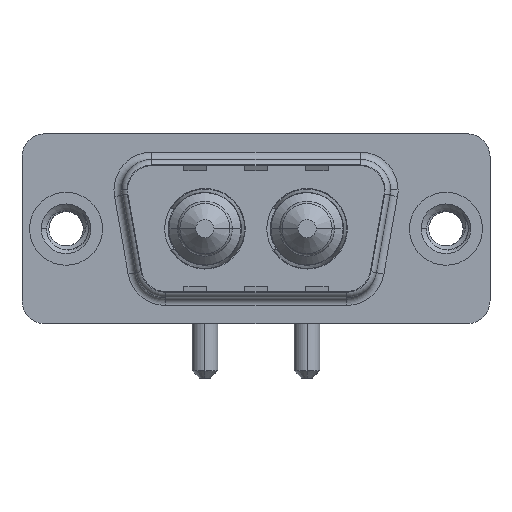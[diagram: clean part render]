
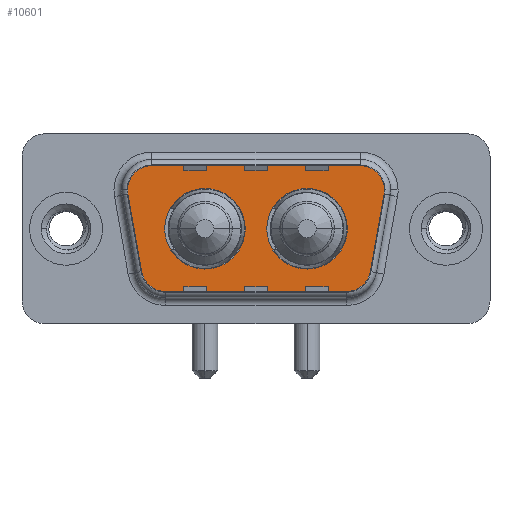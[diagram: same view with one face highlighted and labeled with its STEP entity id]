
A CAD part, top view. The second image highlights one B-rep face of the part: STEP entity #10601.
In plain terms, the highlighted planar face has unit normal (0, 0, 1).
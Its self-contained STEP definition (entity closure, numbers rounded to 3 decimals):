
#121 = EDGE_CURVE ( 'NONE', #11230, #8810, #10595, .T. ) ;
#185 = DIRECTION ( 'NONE',  ( 0., 0., 1. ) ) ;
#381 = DIRECTION ( 'NONE',  ( 0., 0., 1. ) ) ;
#634 = CARTESIAN_POINT ( 'NONE',  ( 21.534, 2.553, 0. ) ) ;
#751 = VECTOR ( 'NONE', #9647, 1000. ) ;
#845 = ORIENTED_EDGE ( 'NONE', *, *, #121, .T. ) ;
#1028 = DIRECTION ( 'NONE',  ( 0., 0., 1. ) ) ;
#1068 = DIRECTION ( 'NONE',  ( 0., 0., 1. ) ) ;
#1150 = FACE_OUTER_BOUND ( 'NONE', #7707, .T. ) ;
#1158 = EDGE_CURVE ( 'NONE', #3391, #4372, #2509, .T. ) ;
#1253 = CARTESIAN_POINT ( 'NONE',  ( 5.436, 4.9, 0. ) ) ;
#1506 = DIRECTION ( 'NONE',  ( 0., 0., 1. ) ) ;
#1563 = CARTESIAN_POINT ( 'NONE',  ( 6.459, -2.9, 0. ) ) ;
#1573 = AXIS2_PLACEMENT_3D ( 'NONE', #2389, #1506, #6002 ) ;
#1911 = PLANE ( 'NONE',  #5977 ) ;
#1923 = EDGE_CURVE ( 'NONE', #4514, #3446, #9788, .T. ) ;
#2010 = EDGE_CURVE ( 'NONE', #5898, #9227, #8078, .T. ) ;
#2159 = CARTESIAN_POINT ( 'NONE',  ( 3.466, 2.553, 0. ) ) ;
#2242 = DIRECTION ( 'NONE',  ( 1., 0., 0. ) ) ;
#2358 = CARTESIAN_POINT ( 'NONE',  ( 9.14, 0., 0. ) ) ;
#2389 = CARTESIAN_POINT ( 'NONE',  ( 5.436, 2.9, 0. ) ) ;
#2408 = CARTESIAN_POINT ( 'NONE',  ( 21.564, 2.9, 0. ) ) ;
#2444 = ORIENTED_EDGE ( 'NONE', *, *, #6426, .T. ) ;
#2509 = LINE ( 'NONE', #634, #9070 ) ;
#2644 = CARTESIAN_POINT ( 'NONE',  ( 20.511, -3.247, 0. ) ) ;
#2742 = ORIENTED_EDGE ( 'NONE', *, *, #4454, .T. ) ;
#2781 = CARTESIAN_POINT ( 'NONE',  ( 3.466, 2.553, 0. ) ) ;
#2819 = CIRCLE ( 'NONE', #6562, 2.65 ) ;
#3036 = DIRECTION ( 'NONE',  ( 0.174, -0.985, 0. ) ) ;
#3181 = DIRECTION ( 'NONE',  ( 1., 0., 0. ) ) ;
#3182 = DIRECTION ( 'NONE',  ( -1., 0., 0. ) ) ;
#3293 = CARTESIAN_POINT ( 'NONE',  ( 18.541, -2.9, 0. ) ) ;
#3391 = VERTEX_POINT ( 'NONE', #2644 ) ;
#3446 = VERTEX_POINT ( 'NONE', #7868 ) ;
#3484 = CARTESIAN_POINT ( 'NONE',  ( 13.21, 0., 0. ) ) ;
#3557 = CIRCLE ( 'NONE', #7702, 2. ) ;
#4012 = CARTESIAN_POINT ( 'NONE',  ( 5.436, 4.9, 0. ) ) ;
#4174 = CARTESIAN_POINT ( 'NONE',  ( 19.564, 2.9, 0. ) ) ;
#4320 = DIRECTION ( 'NONE',  ( -1., 0., 0. ) ) ;
#4372 = VERTEX_POINT ( 'NONE', #6776 ) ;
#4383 = AXIS2_PLACEMENT_3D ( 'NONE', #1563, #1068, #4320 ) ;
#4435 = ORIENTED_EDGE ( 'NONE', *, *, #5691, .F. ) ;
#4448 = ORIENTED_EDGE ( 'NONE', *, *, #1923, .F. ) ;
#4454 = EDGE_CURVE ( 'NONE', #8600, #9421, #6631, .T. ) ;
#4482 = VECTOR ( 'NONE', #3036, 1000. ) ;
#4514 = VERTEX_POINT ( 'NONE', #3484 ) ;
#4700 = AXIS2_PLACEMENT_3D ( 'NONE', #2358, #5804, #2242 ) ;
#4724 = DIRECTION ( 'NONE',  ( 1., 0., 0. ) ) ;
#4771 = VERTEX_POINT ( 'NONE', #6532 ) ;
#4887 = DIRECTION ( 'NONE',  ( -1., 0., 0. ) ) ;
#4957 = LINE ( 'NONE', #2159, #4482 ) ;
#5174 = CARTESIAN_POINT ( 'NONE',  ( 19.564, 2.9, 0. ) ) ;
#5418 = VERTEX_POINT ( 'NONE', #5915 ) ;
#5480 = CARTESIAN_POINT ( 'NONE',  ( 18.541, -2.9, 0. ) ) ;
#5557 = ORIENTED_EDGE ( 'NONE', *, *, #11087, .F. ) ;
#5569 = DIRECTION ( 'NONE',  ( 1., 0., 0. ) ) ;
#5691 = EDGE_CURVE ( 'NONE', #9227, #5898, #7757, .T. ) ;
#5804 = DIRECTION ( 'NONE',  ( 0., 0., 1. ) ) ;
#5850 = CARTESIAN_POINT ( 'NONE',  ( 9.14, 0., 0. ) ) ;
#5898 = VERTEX_POINT ( 'NONE', #6249 ) ;
#5915 = CARTESIAN_POINT ( 'NONE',  ( 6.459, -4.9, 0. ) ) ;
#5937 = ORIENTED_EDGE ( 'NONE', *, *, #10634, .T. ) ;
#5977 = AXIS2_PLACEMENT_3D ( 'NONE', #5480, #1028, #4724 ) ;
#6002 = DIRECTION ( 'NONE',  ( 1., 0., 0. ) ) ;
#6005 = CARTESIAN_POINT ( 'NONE',  ( 11.79, 0., 0. ) ) ;
#6045 = CARTESIAN_POINT ( 'NONE',  ( 6.459, -4.9, 0. ) ) ;
#6171 = DIRECTION ( 'NONE',  ( 0., 0., 1. ) ) ;
#6249 = CARTESIAN_POINT ( 'NONE',  ( 6.49, 0., 0. ) ) ;
#6351 = FACE_BOUND ( 'NONE', #9599, .T. ) ;
#6426 = EDGE_CURVE ( 'NONE', #4771, #5418, #10391, .T. ) ;
#6454 = EDGE_CURVE ( 'NONE', #8810, #8600, #10176, .T. ) ;
#6532 = CARTESIAN_POINT ( 'NONE',  ( 4.489, -3.247, 0. ) ) ;
#6562 = AXIS2_PLACEMENT_3D ( 'NONE', #7341, #185, #5569 ) ;
#6631 = CIRCLE ( 'NONE', #1573, 2. ) ;
#6776 = CARTESIAN_POINT ( 'NONE',  ( 21.534, 2.553, 0. ) ) ;
#6900 = CIRCLE ( 'NONE', #11585, 2. ) ;
#7223 = CARTESIAN_POINT ( 'NONE',  ( 15.86, 0., 0. ) ) ;
#7251 = ORIENTED_EDGE ( 'NONE', *, *, #6454, .T. ) ;
#7341 = CARTESIAN_POINT ( 'NONE',  ( 15.86, 0., 0. ) ) ;
#7610 = CARTESIAN_POINT ( 'NONE',  ( 18.541, -4.9, 0. ) ) ;
#7702 = AXIS2_PLACEMENT_3D ( 'NONE', #3293, #381, #3181 ) ;
#7707 = EDGE_LOOP ( 'NONE', ( #8492, #11196, #10818, #845, #7251, #2742, #5937, #2444, #8847 ) ) ;
#7709 = DIRECTION ( 'NONE',  ( 0., 0., 1. ) ) ;
#7732 = AXIS2_PLACEMENT_3D ( 'NONE', #7223, #6171, #10755 ) ;
#7757 = CIRCLE ( 'NONE', #11485, 2.65 ) ;
#7868 = CARTESIAN_POINT ( 'NONE',  ( 18.51, 0., 0. ) ) ;
#7917 = EDGE_LOOP ( 'NONE', ( #5557, #4448 ) ) ;
#7929 = CARTESIAN_POINT ( 'NONE',  ( 19.564, 4.9, 0. ) ) ;
#8078 = CIRCLE ( 'NONE', #4700, 2.65 ) ;
#8416 = EDGE_CURVE ( 'NONE', #5418, #10606, #9817, .T. ) ;
#8492 = ORIENTED_EDGE ( 'NONE', *, *, #8739, .T. ) ;
#8600 = VERTEX_POINT ( 'NONE', #1253 ) ;
#8726 = AXIS2_PLACEMENT_3D ( 'NONE', #4174, #7709, #3182 ) ;
#8739 = EDGE_CURVE ( 'NONE', #10606, #3391, #3557, .T. ) ;
#8810 = VERTEX_POINT ( 'NONE', #7929 ) ;
#8847 = ORIENTED_EDGE ( 'NONE', *, *, #8416, .T. ) ;
#9070 = VECTOR ( 'NONE', #9598, 1000. ) ;
#9189 = FACE_BOUND ( 'NONE', #7917, .T. ) ;
#9227 = VERTEX_POINT ( 'NONE', #6005 ) ;
#9421 = VERTEX_POINT ( 'NONE', #2781 ) ;
#9598 = DIRECTION ( 'NONE',  ( 0.174, 0.985, 0. ) ) ;
#9599 = EDGE_LOOP ( 'NONE', ( #4435, #10808 ) ) ;
#9647 = DIRECTION ( 'NONE',  ( 1., 0., 0. ) ) ;
#9758 = EDGE_CURVE ( 'NONE', #4372, #11230, #6900, .T. ) ;
#9788 = CIRCLE ( 'NONE', #7732, 2.65 ) ;
#9817 = LINE ( 'NONE', #6045, #751 ) ;
#10176 = LINE ( 'NONE', #4012, #10949 ) ;
#10382 = DIRECTION ( 'NONE',  ( 1., 0., 0. ) ) ;
#10391 = CIRCLE ( 'NONE', #4383, 2. ) ;
#10433 = DIRECTION ( 'NONE',  ( 0., 0., 1. ) ) ;
#10595 = CIRCLE ( 'NONE', #8726, 2. ) ;
#10601 = ADVANCED_FACE ( 'NONE', ( #9189, #6351, #1150 ), #1911, .T. ) ;
#10606 = VERTEX_POINT ( 'NONE', #7610 ) ;
#10634 = EDGE_CURVE ( 'NONE', #9421, #4771, #4957, .T. ) ;
#10637 = DIRECTION ( 'NONE',  ( 0., 0., 1. ) ) ;
#10755 = DIRECTION ( 'NONE',  ( 1., 0., 0. ) ) ;
#10805 = DIRECTION ( 'NONE',  ( -1., 0., 0. ) ) ;
#10808 = ORIENTED_EDGE ( 'NONE', *, *, #2010, .F. ) ;
#10818 = ORIENTED_EDGE ( 'NONE', *, *, #9758, .T. ) ;
#10949 = VECTOR ( 'NONE', #4887, 1000. ) ;
#11087 = EDGE_CURVE ( 'NONE', #3446, #4514, #2819, .T. ) ;
#11196 = ORIENTED_EDGE ( 'NONE', *, *, #1158, .T. ) ;
#11230 = VERTEX_POINT ( 'NONE', #2408 ) ;
#11485 = AXIS2_PLACEMENT_3D ( 'NONE', #5850, #10433, #10382 ) ;
#11585 = AXIS2_PLACEMENT_3D ( 'NONE', #5174, #10637, #10805 ) ;
